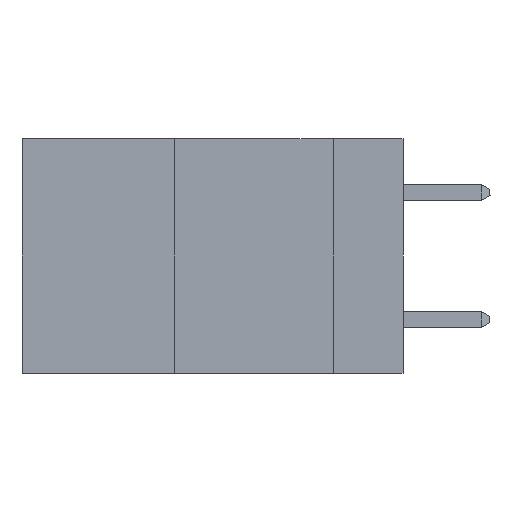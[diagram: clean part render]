
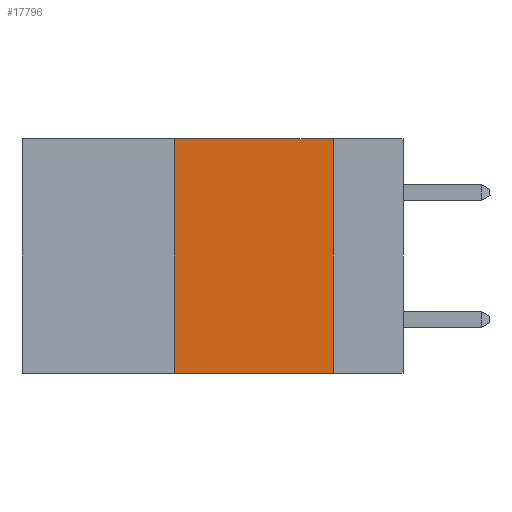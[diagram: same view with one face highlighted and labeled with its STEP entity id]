
A CAD part, left-side view. The second image highlights one B-rep face of the part: STEP entity #17796.
In plain terms, the highlighted planar face has unit normal (-1, 0, 0).
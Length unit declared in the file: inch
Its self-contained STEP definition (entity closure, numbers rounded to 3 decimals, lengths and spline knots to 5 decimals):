
#109 = CARTESIAN_POINT ( 'NONE',  ( 0., 0.11, 0. ) ) ;
#300 = VECTOR ( 'NONE', #19634, 39.37008 ) ;
#1203 = FACE_OUTER_BOUND ( 'NONE', #16322, .T. ) ;
#1653 = CARTESIAN_POINT ( 'NONE',  ( 0., 0.6, -0.37 ) ) ;
#4190 = LINE ( 'NONE', #1653, #28146 ) ;
#4472 = EDGE_CURVE ( 'NONE', #28606, #7970, #24955, .T. ) ;
#5625 = CARTESIAN_POINT ( 'NONE',  ( 0., 0.36, -0.37 ) ) ;
#7970 = VERTEX_POINT ( 'NONE', #20144 ) ;
#9761 = VECTOR ( 'NONE', #30680, 39.37008 ) ;
#11757 = CARTESIAN_POINT ( 'NONE',  ( 0., 0.36, 0. ) ) ;
#14702 = CARTESIAN_POINT ( 'NONE',  ( 0., 0.36, 0. ) ) ;
#15013 = EDGE_CURVE ( 'NONE', #29023, #34978, #22556, .T. ) ;
#15481 = VECTOR ( 'NONE', #30789, 39.37008 ) ;
#15871 = ORIENTED_EDGE ( 'NONE', *, *, #4472, .F. ) ;
#15938 = ORIENTED_EDGE ( 'NONE', *, *, #15013, .F. ) ;
#16322 = EDGE_LOOP ( 'NONE', ( #15871, #17137, #15938, #30280 ) ) ;
#17137 = ORIENTED_EDGE ( 'NONE', *, *, #23113, .F. ) ;
#17261 = AXIS2_PLACEMENT_3D ( 'NONE', #17746, #28697, #18998 ) ;
#17746 = CARTESIAN_POINT ( 'NONE',  ( 0., 0.6, 0. ) ) ;
#17796 = ADVANCED_FACE ( 'NONE', ( #1203 ), #31381, .F. ) ;
#18998 = DIRECTION ( 'NONE',  ( 0., 0., -1. ) ) ;
#19634 = DIRECTION ( 'NONE',  ( 0., -1., 0. ) ) ;
#20144 = CARTESIAN_POINT ( 'NONE',  ( 0., 0.11, -0.37 ) ) ;
#22556 = LINE ( 'NONE', #11757, #15481 ) ;
#23113 = EDGE_CURVE ( 'NONE', #34978, #28606, #25020, .T. ) ;
#23773 = DIRECTION ( 'NONE',  ( 0., -1., 0. ) ) ;
#24843 = CARTESIAN_POINT ( 'NONE',  ( 0., 0.6, 0. ) ) ;
#24955 = LINE ( 'NONE', #27982, #9761 ) ;
#25020 = LINE ( 'NONE', #24843, #300 ) ;
#27914 = EDGE_CURVE ( 'NONE', #29023, #7970, #4190, .T. ) ;
#27982 = CARTESIAN_POINT ( 'NONE',  ( 0., 0.11, 0. ) ) ;
#28146 = VECTOR ( 'NONE', #23773, 39.37008 ) ;
#28606 = VERTEX_POINT ( 'NONE', #109 ) ;
#28697 = DIRECTION ( 'NONE',  ( 1., 0., 0. ) ) ;
#29023 = VERTEX_POINT ( 'NONE', #5625 ) ;
#30280 = ORIENTED_EDGE ( 'NONE', *, *, #27914, .T. ) ;
#30680 = DIRECTION ( 'NONE',  ( 0., 0., -1. ) ) ;
#30789 = DIRECTION ( 'NONE',  ( 0., 0., 1. ) ) ;
#31381 = PLANE ( 'NONE',  #17261 ) ;
#34978 = VERTEX_POINT ( 'NONE', #14702 ) ;
